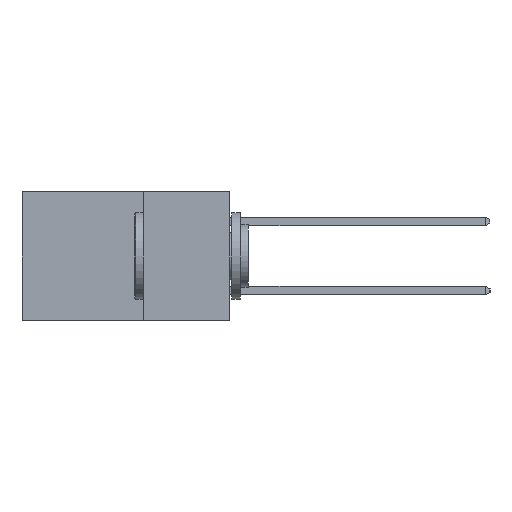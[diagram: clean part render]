
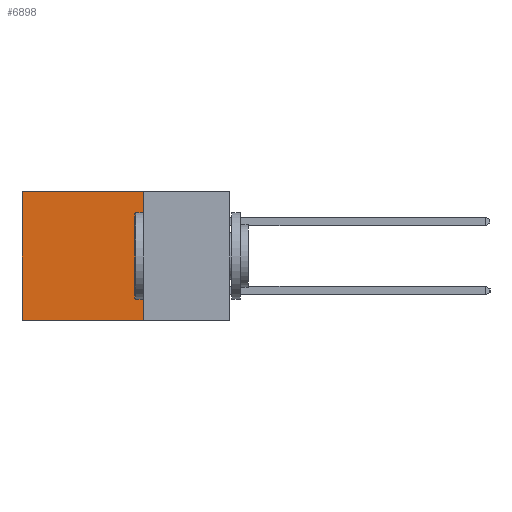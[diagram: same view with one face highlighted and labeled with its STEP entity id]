
A CAD part, left-side view. The second image highlights one B-rep face of the part: STEP entity #6898.
In plain terms, the highlighted planar face has unit normal (-1, 0, 0).
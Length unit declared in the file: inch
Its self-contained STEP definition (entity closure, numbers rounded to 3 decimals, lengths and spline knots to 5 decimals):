
#272 = CARTESIAN_POINT ( 'NONE',  ( 0.2615, 0.6, -0.37 ) ) ;
#326 = LINE ( 'NONE', #7758, #9685 ) ;
#586 = FACE_OUTER_BOUND ( 'NONE', #956, .T. ) ;
#593 = ORIENTED_EDGE ( 'NONE', *, *, #4502, .T. ) ;
#953 = ORIENTED_EDGE ( 'NONE', *, *, #9106, .F. ) ;
#956 = EDGE_LOOP ( 'NONE', ( #593, #953, #1328, #14326 ) ) ;
#1328 = ORIENTED_EDGE ( 'NONE', *, *, #1643, .F. ) ;
#1643 = EDGE_CURVE ( 'NONE', #8458, #6214, #326, .T. ) ;
#1903 = VECTOR ( 'NONE', #10986, 39.37008 ) ;
#2490 = DIRECTION ( 'NONE',  ( 0., 0., -1. ) ) ;
#3220 = AXIS2_PLACEMENT_3D ( 'NONE', #12584, #12164, #12158 ) ;
#3947 = CARTESIAN_POINT ( 'NONE',  ( 0.2615, 0.25, 0. ) ) ;
#4098 = CARTESIAN_POINT ( 'NONE',  ( 0.2615, 0.6, -0.37 ) ) ;
#4502 = EDGE_CURVE ( 'NONE', #10656, #13084, #6451, .T. ) ;
#5523 = LINE ( 'NONE', #3947, #8393 ) ;
#5783 = DIRECTION ( 'NONE',  ( 0., 1., 0. ) ) ;
#6214 = VERTEX_POINT ( 'NONE', #11586 ) ;
#6451 = LINE ( 'NONE', #4098, #9314 ) ;
#6872 = CARTESIAN_POINT ( 'NONE',  ( 0.2615, 0.25, 0. ) ) ;
#6898 = ADVANCED_FACE ( 'NONE', ( #586 ), #12192, .F. ) ;
#7758 = CARTESIAN_POINT ( 'NONE',  ( 0.2615, 0.25, -0.37 ) ) ;
#8393 = VECTOR ( 'NONE', #5783, 39.37008 ) ;
#8458 = VERTEX_POINT ( 'NONE', #6872 ) ;
#9106 = EDGE_CURVE ( 'NONE', #6214, #13084, #11561, .T. ) ;
#9314 = VECTOR ( 'NONE', #11730, 39.37008 ) ;
#9685 = VECTOR ( 'NONE', #2490, 39.37008 ) ;
#10047 = CARTESIAN_POINT ( 'NONE',  ( 0.2615, 0.6, 0. ) ) ;
#10656 = VERTEX_POINT ( 'NONE', #10047 ) ;
#10986 = DIRECTION ( 'NONE',  ( 0., 1., 0. ) ) ;
#11000 = CARTESIAN_POINT ( 'NONE',  ( 0.2615, 0.25, -0.37 ) ) ;
#11561 = LINE ( 'NONE', #11000, #1903 ) ;
#11586 = CARTESIAN_POINT ( 'NONE',  ( 0.2615, 0.25, -0.37 ) ) ;
#11730 = DIRECTION ( 'NONE',  ( 0., 0., -1. ) ) ;
#12158 = DIRECTION ( 'NONE',  ( 0., 0., -1. ) ) ;
#12164 = DIRECTION ( 'NONE',  ( 1., 0., 0. ) ) ;
#12192 = PLANE ( 'NONE',  #3220 ) ;
#12584 = CARTESIAN_POINT ( 'NONE',  ( 0.2615, 0.25, -0.37 ) ) ;
#13084 = VERTEX_POINT ( 'NONE', #272 ) ;
#13269 = EDGE_CURVE ( 'NONE', #8458, #10656, #5523, .T. ) ;
#14326 = ORIENTED_EDGE ( 'NONE', *, *, #13269, .T. ) ;
